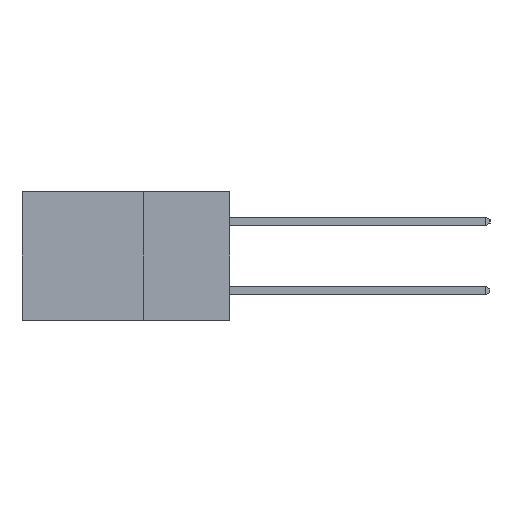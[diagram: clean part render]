
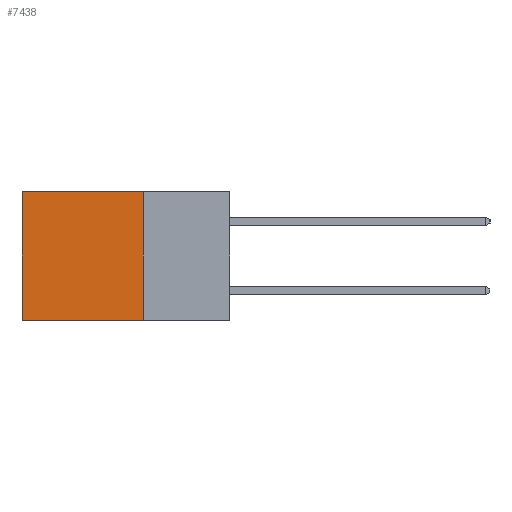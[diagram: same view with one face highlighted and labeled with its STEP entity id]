
A CAD part, left-side view. The second image highlights one B-rep face of the part: STEP entity #7438.
In plain terms, the highlighted planar face has unit normal (-1, 0, 0).
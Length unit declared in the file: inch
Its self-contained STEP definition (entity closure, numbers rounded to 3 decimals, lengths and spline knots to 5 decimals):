
#164 = EDGE_CURVE ( 'NONE', #9316, #8407, #2412, .T. ) ;
#422 = ORIENTED_EDGE ( 'NONE', *, *, #164, .T. ) ;
#571 = EDGE_CURVE ( 'NONE', #16405, #844, #3211, .T. ) ;
#844 = VERTEX_POINT ( 'NONE', #16025 ) ;
#909 = DIRECTION ( 'NONE',  ( 0., 1., 0. ) ) ;
#1000 = DIRECTION ( 'NONE',  ( 0., 0., -1. ) ) ;
#1203 = DIRECTION ( 'NONE',  ( 0., 0., -1. ) ) ;
#1311 = ORIENTED_EDGE ( 'NONE', *, *, #4875, .T. ) ;
#2412 = LINE ( 'NONE', #8379, #8706 ) ;
#2448 = AXIS2_PLACEMENT_3D ( 'NONE', #16380, #8777, #1203 ) ;
#2942 = EDGE_CURVE ( 'NONE', #844, #8407, #9985, .T. ) ;
#3211 = LINE ( 'NONE', #7192, #16247 ) ;
#4659 = CARTESIAN_POINT ( 'NONE',  ( 0.298, 0.25, -0.37 ) ) ;
#4875 = EDGE_CURVE ( 'NONE', #16405, #9316, #15523, .T. ) ;
#4929 = FACE_OUTER_BOUND ( 'NONE', #7012, .T. ) ;
#6644 = VECTOR ( 'NONE', #909, 39.37008 ) ;
#7012 = EDGE_LOOP ( 'NONE', ( #422, #13918, #8601, #1311 ) ) ;
#7192 = CARTESIAN_POINT ( 'NONE',  ( 0.298, 0.25, 0. ) ) ;
#7438 = ADVANCED_FACE ( 'NONE', ( #4929 ), #8724, .F. ) ;
#8379 = CARTESIAN_POINT ( 'NONE',  ( 0.298, 0.6, 0. ) ) ;
#8407 = VERTEX_POINT ( 'NONE', #9354 ) ;
#8601 = ORIENTED_EDGE ( 'NONE', *, *, #571, .F. ) ;
#8706 = VECTOR ( 'NONE', #14734, 39.37008 ) ;
#8724 = PLANE ( 'NONE',  #2448 ) ;
#8777 = DIRECTION ( 'NONE',  ( 1., 0., 0. ) ) ;
#8913 = CARTESIAN_POINT ( 'NONE',  ( 0.298, 0.25, 0. ) ) ;
#9316 = VERTEX_POINT ( 'NONE', #16384 ) ;
#9354 = CARTESIAN_POINT ( 'NONE',  ( 0.298, 0.6, -0.37 ) ) ;
#9832 = DIRECTION ( 'NONE',  ( 0., 1., 0. ) ) ;
#9985 = LINE ( 'NONE', #4659, #6644 ) ;
#12127 = VECTOR ( 'NONE', #9832, 39.37008 ) ;
#12172 = CARTESIAN_POINT ( 'NONE',  ( 0.298, 0.25, 0. ) ) ;
#13918 = ORIENTED_EDGE ( 'NONE', *, *, #2942, .F. ) ;
#14734 = DIRECTION ( 'NONE',  ( 0., 0., -1. ) ) ;
#15523 = LINE ( 'NONE', #8913, #12127 ) ;
#16025 = CARTESIAN_POINT ( 'NONE',  ( 0.298, 0.25, -0.37 ) ) ;
#16247 = VECTOR ( 'NONE', #1000, 39.37008 ) ;
#16380 = CARTESIAN_POINT ( 'NONE',  ( 0.298, 0.25, 0. ) ) ;
#16384 = CARTESIAN_POINT ( 'NONE',  ( 0.298, 0.6, 0. ) ) ;
#16405 = VERTEX_POINT ( 'NONE', #12172 ) ;
